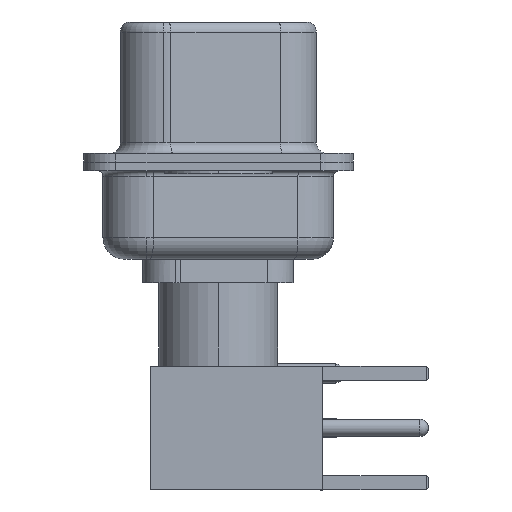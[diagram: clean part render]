
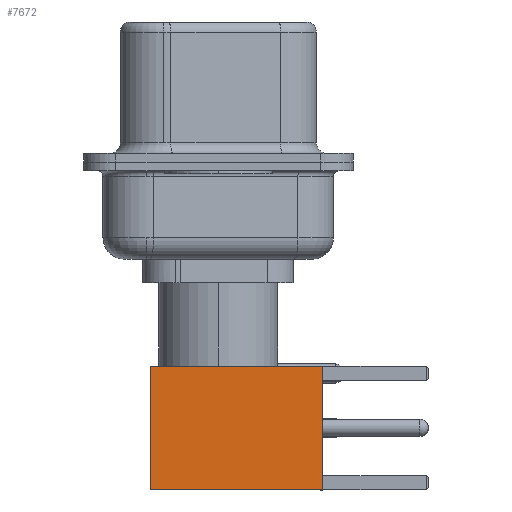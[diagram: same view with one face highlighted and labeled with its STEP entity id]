
A CAD part, left-side view. The second image highlights one B-rep face of the part: STEP entity #7672.
In plain terms, the highlighted face is planar.
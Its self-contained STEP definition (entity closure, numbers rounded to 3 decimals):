
#1311 = VERTEX_POINT ( 'NONE', #23100 ) ;
#1316 = VERTEX_POINT ( 'NONE', #13185 ) ;
#1971 = VERTEX_POINT ( 'NONE', #22475 ) ;
#2556 = DIRECTION ( 'NONE',  ( 0., 0., 1. ) ) ;
#3339 = LINE ( 'NONE', #22277, #7984 ) ;
#3922 = DIRECTION ( 'NONE',  ( 0., 0., -1. ) ) ;
#5379 = ORIENTED_EDGE ( 'NONE', *, *, #23246, .F. ) ;
#5502 = CARTESIAN_POINT ( 'NONE',  ( 2.875, 2.875, 0. ) ) ;
#6086 = ORIENTED_EDGE ( 'NONE', *, *, #21933, .F. ) ;
#7144 = PLANE ( 'NONE',  #15425 ) ;
#7672 = ADVANCED_FACE ( 'NONE', ( #11117 ), #7144, .T. ) ;
#7984 = VECTOR ( 'NONE', #21988, 1000. ) ;
#8061 = CARTESIAN_POINT ( 'NONE',  ( 2.875, 2.875, 8. ) ) ;
#8453 = EDGE_CURVE ( 'NONE', #16894, #1971, #14488, .T. ) ;
#9000 = CARTESIAN_POINT ( 'NONE',  ( 2.875, 2.875, 0. ) ) ;
#9106 = ORIENTED_EDGE ( 'NONE', *, *, #8453, .T. ) ;
#10040 = LINE ( 'NONE', #22787, #17486 ) ;
#11117 = FACE_OUTER_BOUND ( 'NONE', #25314, .T. ) ;
#13185 = CARTESIAN_POINT ( 'NONE',  ( -2.875, 2.875, 8. ) ) ;
#13659 = ORIENTED_EDGE ( 'NONE', *, *, #17412, .T. ) ;
#14184 = DIRECTION ( 'NONE',  ( -1., 0., 0. ) ) ;
#14488 = LINE ( 'NONE', #5502, #25068 ) ;
#14657 = VECTOR ( 'NONE', #22013, 1000. ) ;
#15425 = AXIS2_PLACEMENT_3D ( 'NONE', #9000, #26414, #2556 ) ;
#16894 = VERTEX_POINT ( 'NONE', #8061 ) ;
#17412 = EDGE_CURVE ( 'NONE', #1971, #1311, #3339, .T. ) ;
#17486 = VECTOR ( 'NONE', #14184, 1000. ) ;
#17579 = LINE ( 'NONE', #24286, #14657 ) ;
#21933 = EDGE_CURVE ( 'NONE', #1316, #1311, #17579, .T. ) ;
#21988 = DIRECTION ( 'NONE',  ( -1., 0., 0. ) ) ;
#22013 = DIRECTION ( 'NONE',  ( 0., 0., -1. ) ) ;
#22277 = CARTESIAN_POINT ( 'NONE',  ( 0., 2.875, 0. ) ) ;
#22475 = CARTESIAN_POINT ( 'NONE',  ( 2.875, 2.875, 0. ) ) ;
#22787 = CARTESIAN_POINT ( 'NONE',  ( 0., 2.875, 8. ) ) ;
#23100 = CARTESIAN_POINT ( 'NONE',  ( -2.875, 2.875, 0. ) ) ;
#23246 = EDGE_CURVE ( 'NONE', #16894, #1316, #10040, .T. ) ;
#24286 = CARTESIAN_POINT ( 'NONE',  ( -2.875, 2.875, 0. ) ) ;
#25068 = VECTOR ( 'NONE', #3922, 1000. ) ;
#25314 = EDGE_LOOP ( 'NONE', ( #9106, #13659, #6086, #5379 ) ) ;
#26414 = DIRECTION ( 'NONE',  ( 0., 1., 0. ) ) ;
